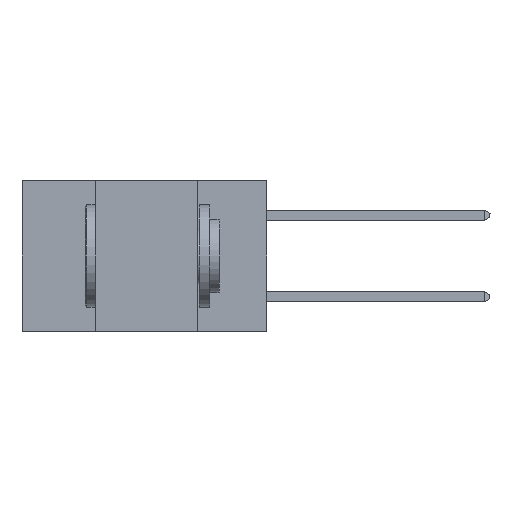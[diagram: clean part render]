
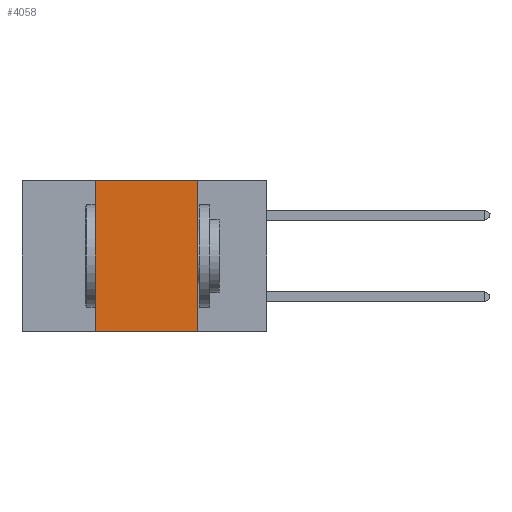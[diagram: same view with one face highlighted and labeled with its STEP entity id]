
A CAD part, left-side view. The second image highlights one B-rep face of the part: STEP entity #4058.
In plain terms, the highlighted planar face has unit normal (-1, 0, 0).
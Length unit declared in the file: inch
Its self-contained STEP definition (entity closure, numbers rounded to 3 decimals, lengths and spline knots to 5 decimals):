
#31 = VERTEX_POINT ( 'NONE', #3040 ) ;
#110 = LINE ( 'NONE', #10137, #6431 ) ;
#516 = DIRECTION ( 'NONE',  ( 0., 0., 1. ) ) ;
#922 = EDGE_CURVE ( 'NONE', #6077, #31, #110, .T. ) ;
#942 = CARTESIAN_POINT ( 'NONE',  ( 0., 0.6, -0.37 ) ) ;
#1135 = VECTOR ( 'NONE', #9067, 39.37008 ) ;
#1746 = DIRECTION ( 'NONE',  ( 1., 0., 0. ) ) ;
#1829 = CARTESIAN_POINT ( 'NONE',  ( 0., 0.42, -0.37 ) ) ;
#1917 = EDGE_CURVE ( 'NONE', #3193, #6077, #11509, .T. ) ;
#2750 = ORIENTED_EDGE ( 'NONE', *, *, #1917, .F. ) ;
#3040 = CARTESIAN_POINT ( 'NONE',  ( 0., 0.17, -0.37 ) ) ;
#3193 = VERTEX_POINT ( 'NONE', #5181 ) ;
#3537 = PLANE ( 'NONE',  #4964 ) ;
#3834 = EDGE_CURVE ( 'NONE', #9549, #3193, #11182, .T. ) ;
#4058 = ADVANCED_FACE ( 'NONE', ( #6636 ), #3537, .F. ) ;
#4218 = ORIENTED_EDGE ( 'NONE', *, *, #3834, .F. ) ;
#4386 = DIRECTION ( 'NONE',  ( 0., -1., 0. ) ) ;
#4445 = CARTESIAN_POINT ( 'NONE',  ( 0., 0.6, 0. ) ) ;
#4464 = CARTESIAN_POINT ( 'NONE',  ( 0., 0.6, 0. ) ) ;
#4565 = VECTOR ( 'NONE', #4386, 39.37008 ) ;
#4785 = CARTESIAN_POINT ( 'NONE',  ( 0., 0.17, 0. ) ) ;
#4916 = CARTESIAN_POINT ( 'NONE',  ( 0., 0.42, 0. ) ) ;
#4964 = AXIS2_PLACEMENT_3D ( 'NONE', #4445, #1746, #10791 ) ;
#5181 = CARTESIAN_POINT ( 'NONE',  ( 0., 0.42, 0. ) ) ;
#5359 = ORIENTED_EDGE ( 'NONE', *, *, #7387, .T. ) ;
#6077 = VERTEX_POINT ( 'NONE', #4785 ) ;
#6431 = VECTOR ( 'NONE', #10936, 39.37008 ) ;
#6636 = FACE_OUTER_BOUND ( 'NONE', #11350, .T. ) ;
#7036 = LINE ( 'NONE', #942, #1135 ) ;
#7387 = EDGE_CURVE ( 'NONE', #9549, #31, #7036, .T. ) ;
#9067 = DIRECTION ( 'NONE',  ( 0., -1., 0. ) ) ;
#9549 = VERTEX_POINT ( 'NONE', #1829 ) ;
#10137 = CARTESIAN_POINT ( 'NONE',  ( 0., 0.17, 0. ) ) ;
#10791 = DIRECTION ( 'NONE',  ( 0., 0., -1. ) ) ;
#10936 = DIRECTION ( 'NONE',  ( 0., 0., -1. ) ) ;
#11037 = ORIENTED_EDGE ( 'NONE', *, *, #922, .F. ) ;
#11182 = LINE ( 'NONE', #4916, #11611 ) ;
#11350 = EDGE_LOOP ( 'NONE', ( #11037, #2750, #4218, #5359 ) ) ;
#11509 = LINE ( 'NONE', #4464, #4565 ) ;
#11611 = VECTOR ( 'NONE', #516, 39.37008 ) ;
